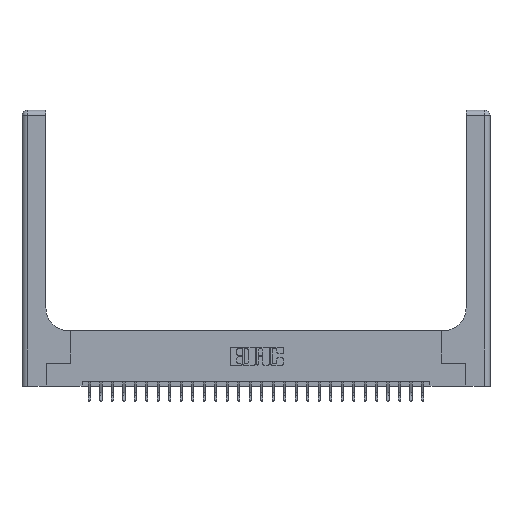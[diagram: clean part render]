
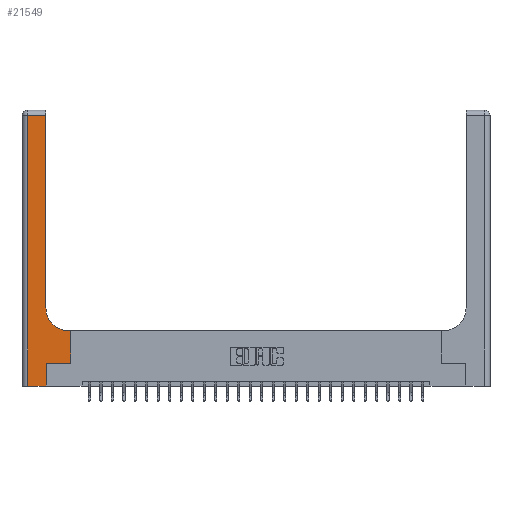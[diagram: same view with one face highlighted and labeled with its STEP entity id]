
A CAD part, top view. The second image highlights one B-rep face of the part: STEP entity #21549.
In plain terms, the highlighted planar face has unit normal (0, 0, 1).
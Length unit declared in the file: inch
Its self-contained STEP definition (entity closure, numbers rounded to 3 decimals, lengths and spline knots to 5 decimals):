
#160 = DIRECTION ( 'NONE',  ( -1., 0., 0. ) ) ;
#305 = VERTEX_POINT ( 'NONE', #9760 ) ;
#810 = VERTEX_POINT ( 'NONE', #7824 ) ;
#920 = VERTEX_POINT ( 'NONE', #23941 ) ;
#1202 = DIRECTION ( 'NONE',  ( -1., 0., 0. ) ) ;
#1626 = LINE ( 'NONE', #15756, #14176 ) ;
#1812 = CARTESIAN_POINT ( 'NONE',  ( 0., 2.94, 0.37 ) ) ;
#2265 = EDGE_CURVE ( 'NONE', #920, #305, #9109, .T. ) ;
#2768 = ORIENTED_EDGE ( 'NONE', *, *, #2265, .T. ) ;
#3972 = DIRECTION ( 'NONE',  ( 1., 0., 0. ) ) ;
#4041 = CARTESIAN_POINT ( 'NONE',  ( 0.528, 0.25, 0.37 ) ) ;
#4339 = ORIENTED_EDGE ( 'NONE', *, *, #5009, .T. ) ;
#4479 = EDGE_CURVE ( 'NONE', #7917, #4619, #1626, .T. ) ;
#4578 = LINE ( 'NONE', #4041, #10043 ) ;
#4619 = VERTEX_POINT ( 'NONE', #23433 ) ;
#5009 = EDGE_CURVE ( 'NONE', #5550, #810, #13176, .T. ) ;
#5550 = VERTEX_POINT ( 'NONE', #21709 ) ;
#6329 = ORIENTED_EDGE ( 'NONE', *, *, #6519, .T. ) ;
#6485 = VERTEX_POINT ( 'NONE', #24207 ) ;
#6519 = EDGE_CURVE ( 'NONE', #810, #19860, #10530, .T. ) ;
#7561 = EDGE_LOOP ( 'NONE', ( #21691, #4339, #6329, #19201, #25146, #14872, #10666, #2768, #9216 ) ) ;
#7824 = CARTESIAN_POINT ( 'NONE',  ( 0.06, 2.94, 0.37 ) ) ;
#7878 = DIRECTION ( 'NONE',  ( -1., 0., 0. ) ) ;
#7917 = VERTEX_POINT ( 'NONE', #21617 ) ;
#8922 = VECTOR ( 'NONE', #3972, 39.37008 ) ;
#9109 = LINE ( 'NONE', #10387, #9419 ) ;
#9216 = ORIENTED_EDGE ( 'NONE', *, *, #20663, .T. ) ;
#9419 = VECTOR ( 'NONE', #160, 39.37008 ) ;
#9760 = CARTESIAN_POINT ( 'NONE',  ( 0.51, 0.6, 0.37 ) ) ;
#9951 = DIRECTION ( 'NONE',  ( 0., 1., 0. ) ) ;
#10043 = VECTOR ( 'NONE', #9951, 39.37008 ) ;
#10387 = CARTESIAN_POINT ( 'NONE',  ( 0.26, 0.6, 0.37 ) ) ;
#10530 = LINE ( 'NONE', #12815, #18585 ) ;
#10552 = FACE_OUTER_BOUND ( 'NONE', #7561, .T. ) ;
#10666 = ORIENTED_EDGE ( 'NONE', *, *, #17317, .T. ) ;
#11519 = LINE ( 'NONE', #24347, #8922 ) ;
#11919 = VECTOR ( 'NONE', #25503, 39.37008 ) ;
#12213 = CIRCLE ( 'NONE', #14816, 0.25 ) ;
#12749 = CARTESIAN_POINT ( 'NONE',  ( 0.26, 3., 0.37 ) ) ;
#12815 = CARTESIAN_POINT ( 'NONE',  ( 0.06, 3., 0.37 ) ) ;
#13176 = LINE ( 'NONE', #1812, #19542 ) ;
#14176 = VECTOR ( 'NONE', #25829, 39.37008 ) ;
#14212 = CARTESIAN_POINT ( 'NONE',  ( 0.06, 0., 0.37 ) ) ;
#14816 = AXIS2_PLACEMENT_3D ( 'NONE', #21414, #25209, #17025 ) ;
#14872 = ORIENTED_EDGE ( 'NONE', *, *, #21701, .T. ) ;
#14988 = CARTESIAN_POINT ( 'NONE',  ( 0., 0., 0.37 ) ) ;
#15676 = AXIS2_PLACEMENT_3D ( 'NONE', #23902, #23723, #1202 ) ;
#15756 = CARTESIAN_POINT ( 'NONE',  ( 0.265, 0., 0.37 ) ) ;
#15885 = EDGE_CURVE ( 'NONE', #18625, #5550, #19747, .T. ) ;
#17025 = DIRECTION ( 'NONE',  ( 1., 0., 0. ) ) ;
#17317 = EDGE_CURVE ( 'NONE', #6485, #920, #4578, .T. ) ;
#17705 = PLANE ( 'NONE',  #15676 ) ;
#18585 = VECTOR ( 'NONE', #19156, 39.37008 ) ;
#18625 = VERTEX_POINT ( 'NONE', #22806 ) ;
#19156 = DIRECTION ( 'NONE',  ( 0., -1., 0. ) ) ;
#19201 = ORIENTED_EDGE ( 'NONE', *, *, #20218, .T. ) ;
#19270 = LINE ( 'NONE', #14988, #11919 ) ;
#19542 = VECTOR ( 'NONE', #7878, 39.37008 ) ;
#19747 = LINE ( 'NONE', #12749, #24927 ) ;
#19860 = VERTEX_POINT ( 'NONE', #14212 ) ;
#20218 = EDGE_CURVE ( 'NONE', #19860, #7917, #19270, .T. ) ;
#20663 = EDGE_CURVE ( 'NONE', #305, #18625, #12213, .T. ) ;
#20998 = DIRECTION ( 'NONE',  ( 0., 1., 0. ) ) ;
#21414 = CARTESIAN_POINT ( 'NONE',  ( 0.51, 0.85, 0.37 ) ) ;
#21549 = ADVANCED_FACE ( 'NONE', ( #10552 ), #17705, .F. ) ;
#21617 = CARTESIAN_POINT ( 'NONE',  ( 0.265, 0., 0.37 ) ) ;
#21691 = ORIENTED_EDGE ( 'NONE', *, *, #15885, .T. ) ;
#21701 = EDGE_CURVE ( 'NONE', #4619, #6485, #11519, .T. ) ;
#21709 = CARTESIAN_POINT ( 'NONE',  ( 0.26, 2.94, 0.37 ) ) ;
#22806 = CARTESIAN_POINT ( 'NONE',  ( 0.26, 0.85, 0.37 ) ) ;
#23433 = CARTESIAN_POINT ( 'NONE',  ( 0.265, 0.25, 0.37 ) ) ;
#23723 = DIRECTION ( 'NONE',  ( 0., 0., -1. ) ) ;
#23902 = CARTESIAN_POINT ( 'NONE',  ( 0., 3., 0.37 ) ) ;
#23941 = CARTESIAN_POINT ( 'NONE',  ( 0.528, 0.6, 0.37 ) ) ;
#24207 = CARTESIAN_POINT ( 'NONE',  ( 0.528, 0.25, 0.37 ) ) ;
#24347 = CARTESIAN_POINT ( 'NONE',  ( 0.265, 0.25, 0.37 ) ) ;
#24927 = VECTOR ( 'NONE', #20998, 39.37008 ) ;
#25146 = ORIENTED_EDGE ( 'NONE', *, *, #4479, .T. ) ;
#25209 = DIRECTION ( 'NONE',  ( 0., 0., -1. ) ) ;
#25503 = DIRECTION ( 'NONE',  ( 1., 0., 0. ) ) ;
#25829 = DIRECTION ( 'NONE',  ( 0., 1., 0. ) ) ;
